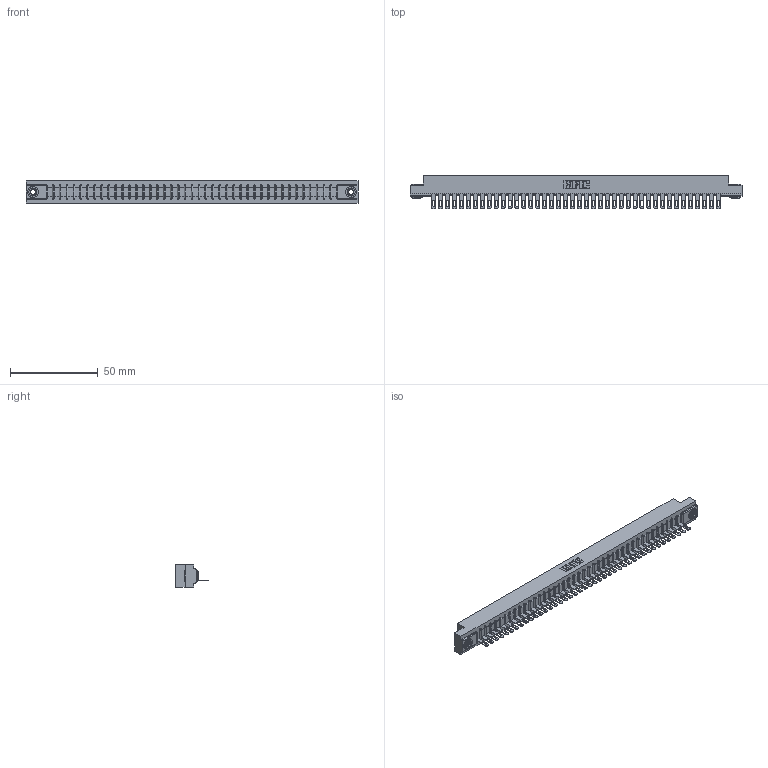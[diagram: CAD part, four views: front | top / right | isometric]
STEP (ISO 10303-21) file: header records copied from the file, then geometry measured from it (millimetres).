
FILE_DESCRIPTION (( 'STEP AP203' ), '1' );
FILE_NAME ('307-042-505-103.STEP', '2019-09-04T07:27:56', ( '' ), ( '' ), 'SwSTEP 2.0', 'SolidWorks 2016', '' );
FILE_SCHEMA (( 'CONFIG_CONTROL_DESIGN' ));
Length unit declared in the file: inch
Products named in the file (4): 307-290-001_505; 307-042-505-103; 345-250-002_345-250-002-102; 307 Part_.156 Dia Mounting Holes
Assembly tree (45 placements, depth 2):
  307-042-505-103
    307 Part_.156 Dia Mounting Holes
    307-290-001_505  x42
    345-250-002_345-250-002-102  x2
Bounding box: 189.43 x 19.18 x 12.7 mm (x, y, z)
Volume: 19723.7 mm3; surface area: 21494.6 mm2
Topology: 45 solids, 45 shells, 2565 faces, 7239 edges, 4650 vertices
Faces by surface type: plane 1606, cylinder 865, sphere 86, cone 8
Entity records: 37045 total; most frequent: CARTESIAN_POINT 6217, ORIENTED_EDGE 6194, DIRECTION 6063, EDGE_CURVE 3097, LINE 2367, VECTOR 2367, VERTEX_POINT 2002, AXIS2_PLACEMENT_3D 1848
